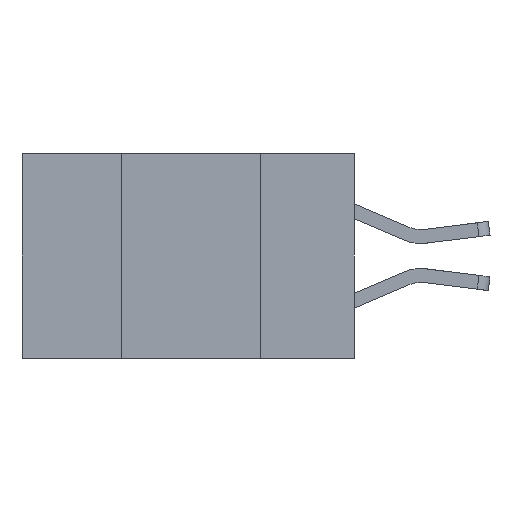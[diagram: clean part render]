
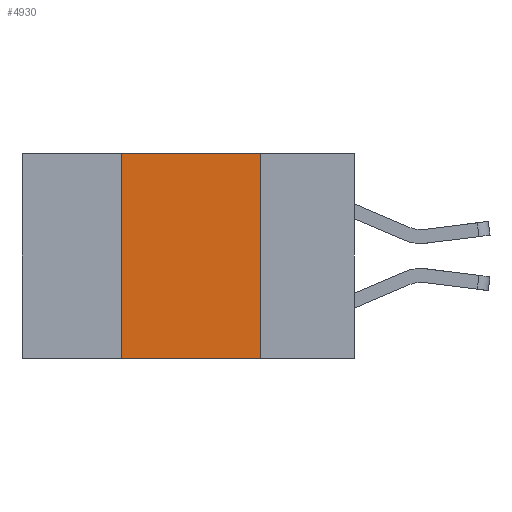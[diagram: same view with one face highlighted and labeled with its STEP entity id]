
A CAD part, left-side view. The second image highlights one B-rep face of the part: STEP entity #4930.
In plain terms, the highlighted planar face has unit normal (-1, 0, 0).
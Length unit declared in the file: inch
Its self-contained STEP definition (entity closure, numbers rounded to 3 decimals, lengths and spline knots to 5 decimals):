
#134 = ORIENTED_EDGE ( 'NONE', *, *, #4706, .F. ) ;
#179 = EDGE_LOOP ( 'NONE', ( #134, #2161, #10015, #1445 ) ) ;
#275 = LINE ( 'NONE', #4271, #4336 ) ;
#314 = CARTESIAN_POINT ( 'NONE',  ( 0., 0.6, 0. ) ) ;
#479 = CARTESIAN_POINT ( 'NONE',  ( 0., 0.6, -0.37 ) ) ;
#552 = VECTOR ( 'NONE', #931, 39.37008 ) ;
#931 = DIRECTION ( 'NONE',  ( 0., 0., -1. ) ) ;
#1134 = FACE_OUTER_BOUND ( 'NONE', #179, .T. ) ;
#1238 = DIRECTION ( 'NONE',  ( 0., -1., 0. ) ) ;
#1445 = ORIENTED_EDGE ( 'NONE', *, *, #1960, .T. ) ;
#1686 = DIRECTION ( 'NONE',  ( 0., -1., 0. ) ) ;
#1927 = LINE ( 'NONE', #479, #4349 ) ;
#1939 = VECTOR ( 'NONE', #5913, 39.37008 ) ;
#1960 = EDGE_CURVE ( 'NONE', #4464, #7956, #1927, .T. ) ;
#2080 = CARTESIAN_POINT ( 'NONE',  ( 0., 0.42, 0. ) ) ;
#2161 = ORIENTED_EDGE ( 'NONE', *, *, #3094, .F. ) ;
#2448 = LINE ( 'NONE', #3326, #552 ) ;
#2733 = CARTESIAN_POINT ( 'NONE',  ( 0., 0.17, 0. ) ) ;
#3094 = EDGE_CURVE ( 'NONE', #9083, #8055, #275, .T. ) ;
#3326 = CARTESIAN_POINT ( 'NONE',  ( 0., 0.17, -0.37 ) ) ;
#4092 = CARTESIAN_POINT ( 'NONE',  ( 0., 0.17, -0.37 ) ) ;
#4271 = CARTESIAN_POINT ( 'NONE',  ( 0., 0.6, 0. ) ) ;
#4309 = DIRECTION ( 'NONE',  ( 1., 0., 0. ) ) ;
#4336 = VECTOR ( 'NONE', #1686, 39.37008 ) ;
#4349 = VECTOR ( 'NONE', #1238, 39.37008 ) ;
#4464 = VERTEX_POINT ( 'NONE', #6819 ) ;
#4706 = EDGE_CURVE ( 'NONE', #8055, #7956, #2448, .T. ) ;
#4930 = ADVANCED_FACE ( 'NONE', ( #1134 ), #7389, .F. ) ;
#5913 = DIRECTION ( 'NONE',  ( 0., 0., 1. ) ) ;
#6610 = DIRECTION ( 'NONE',  ( 0., 0., -1. ) ) ;
#6819 = CARTESIAN_POINT ( 'NONE',  ( 0., 0.42, -0.37 ) ) ;
#7389 = PLANE ( 'NONE',  #8797 ) ;
#7956 = VERTEX_POINT ( 'NONE', #4092 ) ;
#7994 = EDGE_CURVE ( 'NONE', #4464, #9083, #9159, .T. ) ;
#8055 = VERTEX_POINT ( 'NONE', #2733 ) ;
#8797 = AXIS2_PLACEMENT_3D ( 'NONE', #314, #4309, #6610 ) ;
#9083 = VERTEX_POINT ( 'NONE', #2080 ) ;
#9159 = LINE ( 'NONE', #9831, #1939 ) ;
#9831 = CARTESIAN_POINT ( 'NONE',  ( 0., 0.42, -0.37 ) ) ;
#10015 = ORIENTED_EDGE ( 'NONE', *, *, #7994, .F. ) ;
